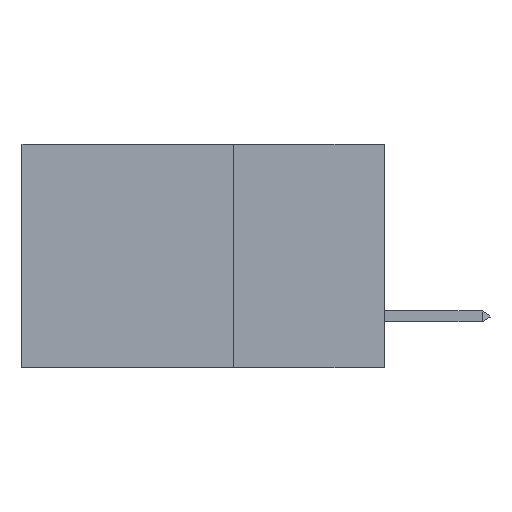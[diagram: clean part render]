
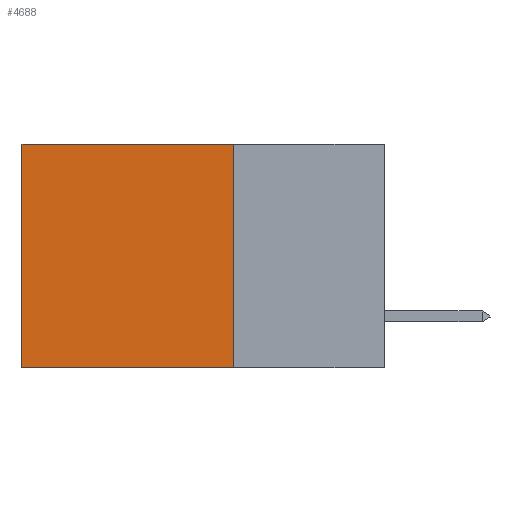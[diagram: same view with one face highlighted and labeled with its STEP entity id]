
A CAD part, left-side view. The second image highlights one B-rep face of the part: STEP entity #4688.
In plain terms, the highlighted planar face has unit normal (-1, 0, 0).
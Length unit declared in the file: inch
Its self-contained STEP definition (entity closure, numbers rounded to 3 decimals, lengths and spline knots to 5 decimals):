
#162 = CARTESIAN_POINT ( 'NONE',  ( 0.2875, 0.25, 0. ) ) ;
#377 = DIRECTION ( 'NONE',  ( 0., 0., -1. ) ) ;
#1314 = EDGE_CURVE ( 'NONE', #8505, #13030, #1949, .T. ) ;
#1675 = LINE ( 'NONE', #12131, #9519 ) ;
#1949 = LINE ( 'NONE', #162, #10328 ) ;
#2530 = DIRECTION ( 'NONE',  ( 0., 1., 0. ) ) ;
#2562 = CARTESIAN_POINT ( 'NONE',  ( 0.2875, 0.25, 0. ) ) ;
#3078 = DIRECTION ( 'NONE',  ( 0., 1., 0. ) ) ;
#3689 = LINE ( 'NONE', #10486, #3868 ) ;
#3868 = VECTOR ( 'NONE', #11698, 39.37008 ) ;
#4688 = ADVANCED_FACE ( 'NONE', ( #13723 ), #11430, .F. ) ;
#5393 = CARTESIAN_POINT ( 'NONE',  ( 0.2875, 0.6, -0.37 ) ) ;
#5886 = EDGE_CURVE ( 'NONE', #13030, #11910, #12289, .T. ) ;
#5960 = VERTEX_POINT ( 'NONE', #11735 ) ;
#7087 = DIRECTION ( 'NONE',  ( 1., 0., 0. ) ) ;
#7263 = CARTESIAN_POINT ( 'NONE',  ( 0.2875, 0.25, 0. ) ) ;
#7358 = ORIENTED_EDGE ( 'NONE', *, *, #5886, .F. ) ;
#7658 = EDGE_LOOP ( 'NONE', ( #10630, #7358, #11441, #10953 ) ) ;
#8505 = VERTEX_POINT ( 'NONE', #7263 ) ;
#8682 = CARTESIAN_POINT ( 'NONE',  ( 0.2875, 0.25, -0.37 ) ) ;
#9519 = VECTOR ( 'NONE', #3078, 39.37008 ) ;
#9592 = EDGE_CURVE ( 'NONE', #8505, #5960, #1675, .T. ) ;
#10213 = AXIS2_PLACEMENT_3D ( 'NONE', #2562, #7087, #377 ) ;
#10328 = VECTOR ( 'NONE', #11376, 39.37008 ) ;
#10486 = CARTESIAN_POINT ( 'NONE',  ( 0.2875, 0.6, 0. ) ) ;
#10529 = VECTOR ( 'NONE', #2530, 39.37008 ) ;
#10630 = ORIENTED_EDGE ( 'NONE', *, *, #12341, .T. ) ;
#10953 = ORIENTED_EDGE ( 'NONE', *, *, #9592, .T. ) ;
#11376 = DIRECTION ( 'NONE',  ( 0., 0., -1. ) ) ;
#11430 = PLANE ( 'NONE',  #10213 ) ;
#11441 = ORIENTED_EDGE ( 'NONE', *, *, #1314, .F. ) ;
#11698 = DIRECTION ( 'NONE',  ( 0., 0., -1. ) ) ;
#11735 = CARTESIAN_POINT ( 'NONE',  ( 0.2875, 0.6, 0. ) ) ;
#11910 = VERTEX_POINT ( 'NONE', #5393 ) ;
#12131 = CARTESIAN_POINT ( 'NONE',  ( 0.2875, 0.25, 0. ) ) ;
#12289 = LINE ( 'NONE', #13649, #10529 ) ;
#12341 = EDGE_CURVE ( 'NONE', #5960, #11910, #3689, .T. ) ;
#13030 = VERTEX_POINT ( 'NONE', #8682 ) ;
#13649 = CARTESIAN_POINT ( 'NONE',  ( 0.2875, 0.25, -0.37 ) ) ;
#13723 = FACE_OUTER_BOUND ( 'NONE', #7658, .T. ) ;
